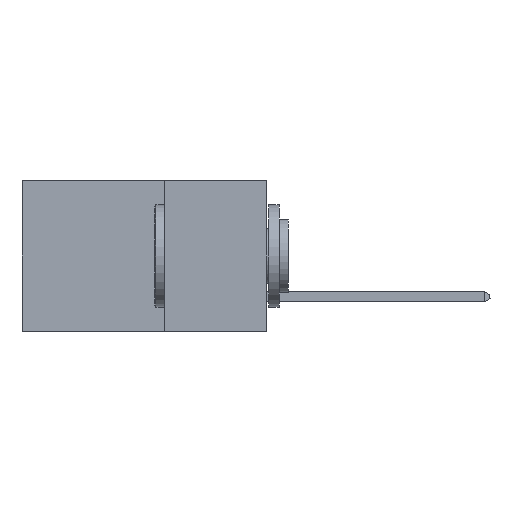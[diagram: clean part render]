
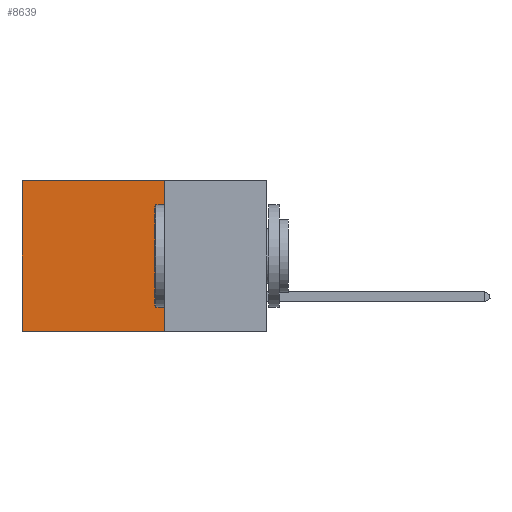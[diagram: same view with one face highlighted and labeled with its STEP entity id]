
A CAD part, left-side view. The second image highlights one B-rep face of the part: STEP entity #8639.
In plain terms, the highlighted planar face has unit normal (-1, 0, 0).
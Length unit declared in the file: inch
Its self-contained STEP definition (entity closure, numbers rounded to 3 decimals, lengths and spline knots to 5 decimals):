
#1230 = ORIENTED_EDGE ( 'NONE', *, *, #22366, .F. ) ;
#3146 = DIRECTION ( 'NONE',  ( 0., 1., 0. ) ) ;
#3570 = LINE ( 'NONE', #17458, #34299 ) ;
#5666 = CARTESIAN_POINT ( 'NONE',  ( 0.2875, 0.25, 0. ) ) ;
#5727 = CARTESIAN_POINT ( 'NONE',  ( 0.2875, 0.25, -0.37 ) ) ;
#6003 = CARTESIAN_POINT ( 'NONE',  ( 0.2875, 0.25, 0. ) ) ;
#6707 = DIRECTION ( 'NONE',  ( 0., 0., -1. ) ) ;
#7387 = CARTESIAN_POINT ( 'NONE',  ( 0.2875, 0.25, -0.37 ) ) ;
#8639 = ADVANCED_FACE ( 'NONE', ( #20831 ), #23394, .F. ) ;
#10056 = EDGE_CURVE ( 'NONE', #25631, #20368, #30493, .T. ) ;
#10209 = CARTESIAN_POINT ( 'NONE',  ( 0.2875, 0.6, -0.37 ) ) ;
#12281 = DIRECTION ( 'NONE',  ( 0., 0., -1. ) ) ;
#12755 = CARTESIAN_POINT ( 'NONE',  ( 0.2875, 0.25, 0. ) ) ;
#12982 = DIRECTION ( 'NONE',  ( 0., 1., 0. ) ) ;
#14094 = VERTEX_POINT ( 'NONE', #6003 ) ;
#14180 = EDGE_CURVE ( 'NONE', #14094, #22136, #23776, .T. ) ;
#15307 = DIRECTION ( 'NONE',  ( 1., 0., 0. ) ) ;
#17458 = CARTESIAN_POINT ( 'NONE',  ( 0.2875, 0.25, 0. ) ) ;
#17482 = AXIS2_PLACEMENT_3D ( 'NONE', #12755, #15307, #12281 ) ;
#18534 = VECTOR ( 'NONE', #22498, 39.37008 ) ;
#19991 = EDGE_LOOP ( 'NONE', ( #35321, #31886, #1230, #26314 ) ) ;
#20368 = VERTEX_POINT ( 'NONE', #10209 ) ;
#20831 = FACE_OUTER_BOUND ( 'NONE', #19991, .T. ) ;
#21861 = EDGE_CURVE ( 'NONE', #22136, #20368, #25780, .T. ) ;
#22136 = VERTEX_POINT ( 'NONE', #32905 ) ;
#22366 = EDGE_CURVE ( 'NONE', #14094, #25631, #3570, .T. ) ;
#22498 = DIRECTION ( 'NONE',  ( 0., 0., -1. ) ) ;
#23244 = VECTOR ( 'NONE', #12982, 39.37008 ) ;
#23394 = PLANE ( 'NONE',  #17482 ) ;
#23776 = LINE ( 'NONE', #5666, #32766 ) ;
#25631 = VERTEX_POINT ( 'NONE', #5727 ) ;
#25780 = LINE ( 'NONE', #30370, #18534 ) ;
#26314 = ORIENTED_EDGE ( 'NONE', *, *, #14180, .T. ) ;
#30370 = CARTESIAN_POINT ( 'NONE',  ( 0.2875, 0.6, 0. ) ) ;
#30493 = LINE ( 'NONE', #7387, #23244 ) ;
#31886 = ORIENTED_EDGE ( 'NONE', *, *, #10056, .F. ) ;
#32766 = VECTOR ( 'NONE', #3146, 39.37008 ) ;
#32905 = CARTESIAN_POINT ( 'NONE',  ( 0.2875, 0.6, 0. ) ) ;
#34299 = VECTOR ( 'NONE', #6707, 39.37008 ) ;
#35321 = ORIENTED_EDGE ( 'NONE', *, *, #21861, .T. ) ;
